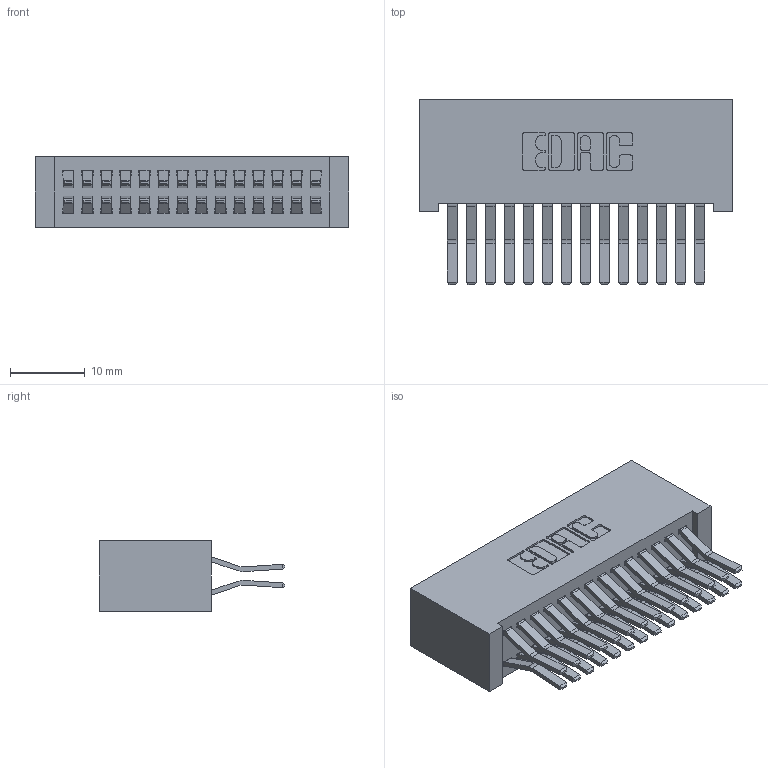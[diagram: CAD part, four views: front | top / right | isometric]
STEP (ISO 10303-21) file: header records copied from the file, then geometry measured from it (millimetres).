
FILE_DESCRIPTION (( 'STEP AP203' ), '1' );
FILE_NAME ('342-028-560-201.STEP', '2018-08-11T14:37:14', ( '' ), ( '' ), 'SwSTEP 2.0', 'SolidWorks 2016', '' );
FILE_SCHEMA (( 'CONFIG_CONTROL_DESIGN' ));
Length unit declared in the file: inch
Products named in the file (3): 345-292-001_560 Tail; 342-028-560-201; 342 Part_Lugless
Assembly tree (29 placements, depth 2):
  342-028-560-201
    342 Part_Lugless
    345-292-001_560 Tail  x28
Bounding box: 41.81 x 24.78 x 9.4 mm (x, y, z)
Volume: 4247.3 mm3; surface area: 7110.6 mm2
Topology: 29 solids, 29 shells, 1614 faces, 4783 edges, 3150 vertices
Faces by surface type: plane 1070, cylinder 544
Entity records: 12307 total; most frequent: CARTESIAN_POINT 2070, ORIENTED_EDGE 2006, DIRECTION 1815, EDGE_CURVE 1003, LINE 879, VECTOR 879, VERTEX_POINT 666, AXIS2_PLACEMENT_3D 468
